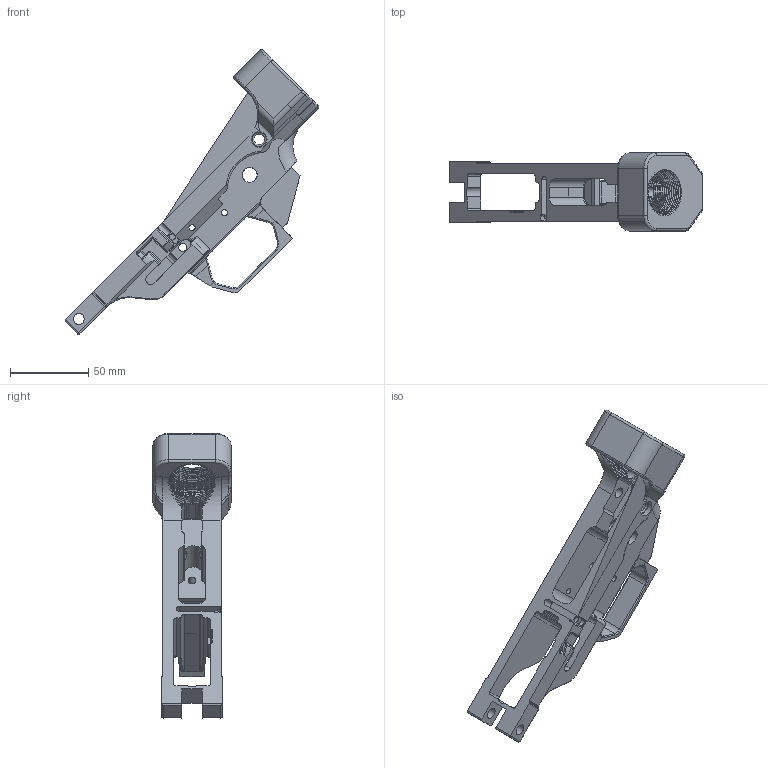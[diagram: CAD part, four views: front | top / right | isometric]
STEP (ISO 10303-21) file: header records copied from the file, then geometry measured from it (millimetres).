
FILE_DESCRIPTION(('Based on JT-Vanguard and Phobos designs for FOSSCAD community. '),'2;1');
FILE_NAME('ArmaDelite_AL-84_Ambi.stp','2015-01-03T15:30:12',('ArmaDelite December 30, 2014'),('FOSSCAD'),'Autodesk Inventor 2013','Autodesk Inventor 2013','');
FILE_SCHEMA(('AUTOMOTIVE_DESIGN { 1 0 10303 214 1 1 1 1 }'));
Length unit declared in the file: millimetre
Products named in the file (1): ArmaDelite_AL-84_Ambi
Bounding box: 162.51 x 50 x 182.34 mm (x, y, z)
Volume: 141327 mm3; surface area: 51346.7 mm2
Topology: 1 solids, 1 shells, 553 faces, 1636 edges, 1073 vertices
Faces by surface type: cylinder 221, plane 178, bspline 87, torus 43, cone 16, sphere 8
Full cylindrical faces by diameter (mm): 2.362 x2, 3.175 x1, 3.969 x5, 5.105 x1, 5.182 x1, 6.477 x1, 6.858 x2, 7 x2, 7.938 x1, 9.525 x2, 10 x1
Entity records: 34184 total; most frequent: CARTESIAN_POINT 19665, ORIENTED_EDGE 3200, DIRECTION 2593, EDGE_CURVE 1600, VERTEX_POINT 1064, AXIS2_PLACEMENT_3D 966, VECTOR 661, LINE 661
